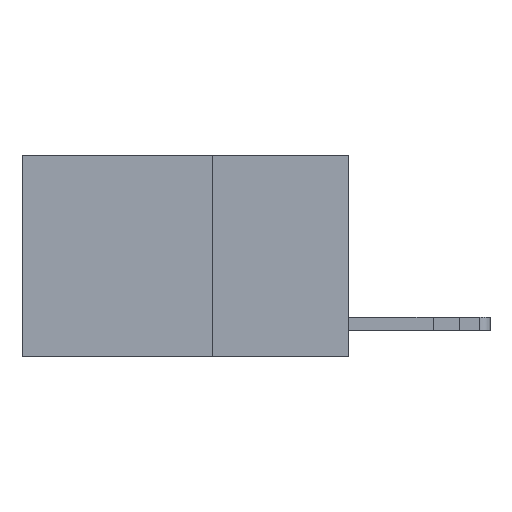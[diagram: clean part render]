
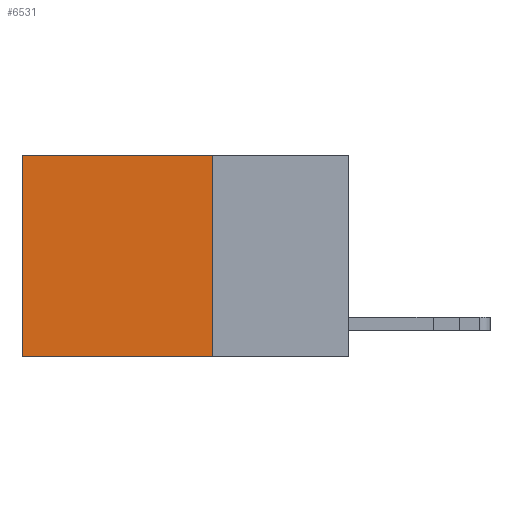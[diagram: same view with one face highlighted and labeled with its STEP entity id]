
A CAD part, left-side view. The second image highlights one B-rep face of the part: STEP entity #6531.
In plain terms, the highlighted planar face has unit normal (-1, 0, 0).
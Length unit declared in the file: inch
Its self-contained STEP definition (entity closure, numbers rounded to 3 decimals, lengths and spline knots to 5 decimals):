
#442 = PLANE ( 'NONE',  #5806 ) ;
#516 = DIRECTION ( 'NONE',  ( 1., 0., 0. ) ) ;
#1535 = EDGE_LOOP ( 'NONE', ( #2408, #4238, #9163, #2842 ) ) ;
#1548 = DIRECTION ( 'NONE',  ( 0., 1., 0. ) ) ;
#2145 = EDGE_CURVE ( 'NONE', #6522, #7753, #4371, .T. ) ;
#2187 = CARTESIAN_POINT ( 'NONE',  ( 0.2625, 0.6, 0. ) ) ;
#2408 = ORIENTED_EDGE ( 'NONE', *, *, #3636, .T. ) ;
#2842 = ORIENTED_EDGE ( 'NONE', *, *, #2145, .T. ) ;
#3097 = FACE_OUTER_BOUND ( 'NONE', #1535, .T. ) ;
#3636 = EDGE_CURVE ( 'NONE', #7753, #5965, #4478, .T. ) ;
#3900 = VECTOR ( 'NONE', #1548, 39.37008 ) ;
#4148 = CARTESIAN_POINT ( 'NONE',  ( 0.2625, 0.6, -0.37 ) ) ;
#4238 = ORIENTED_EDGE ( 'NONE', *, *, #4488, .F. ) ;
#4371 = LINE ( 'NONE', #8036, #11146 ) ;
#4478 = LINE ( 'NONE', #2187, #11249 ) ;
#4488 = EDGE_CURVE ( 'NONE', #8328, #5965, #6540, .T. ) ;
#4817 = DIRECTION ( 'NONE',  ( 0., 0., -1. ) ) ;
#5806 = AXIS2_PLACEMENT_3D ( 'NONE', #9332, #516, #6695 ) ;
#5927 = CARTESIAN_POINT ( 'NONE',  ( 0.2625, 0.25, -0.37 ) ) ;
#5965 = VERTEX_POINT ( 'NONE', #4148 ) ;
#6122 = LINE ( 'NONE', #9237, #8209 ) ;
#6522 = VERTEX_POINT ( 'NONE', #6658 ) ;
#6531 = ADVANCED_FACE ( 'NONE', ( #3097 ), #442, .F. ) ;
#6540 = LINE ( 'NONE', #5927, #3900 ) ;
#6658 = CARTESIAN_POINT ( 'NONE',  ( 0.2625, 0.25, 0. ) ) ;
#6695 = DIRECTION ( 'NONE',  ( 0., 0., -1. ) ) ;
#7138 = EDGE_CURVE ( 'NONE', #6522, #8328, #6122, .T. ) ;
#7753 = VERTEX_POINT ( 'NONE', #9225 ) ;
#8036 = CARTESIAN_POINT ( 'NONE',  ( 0.2625, 0.25, 0. ) ) ;
#8080 = CARTESIAN_POINT ( 'NONE',  ( 0.2625, 0.25, -0.37 ) ) ;
#8209 = VECTOR ( 'NONE', #4817, 39.37008 ) ;
#8328 = VERTEX_POINT ( 'NONE', #8080 ) ;
#8912 = DIRECTION ( 'NONE',  ( 0., 1., 0. ) ) ;
#9163 = ORIENTED_EDGE ( 'NONE', *, *, #7138, .F. ) ;
#9225 = CARTESIAN_POINT ( 'NONE',  ( 0.2625, 0.6, 0. ) ) ;
#9237 = CARTESIAN_POINT ( 'NONE',  ( 0.2625, 0.25, 0. ) ) ;
#9267 = DIRECTION ( 'NONE',  ( 0., 0., -1. ) ) ;
#9332 = CARTESIAN_POINT ( 'NONE',  ( 0.2625, 0.25, 0. ) ) ;
#11146 = VECTOR ( 'NONE', #8912, 39.37008 ) ;
#11249 = VECTOR ( 'NONE', #9267, 39.37008 ) ;
